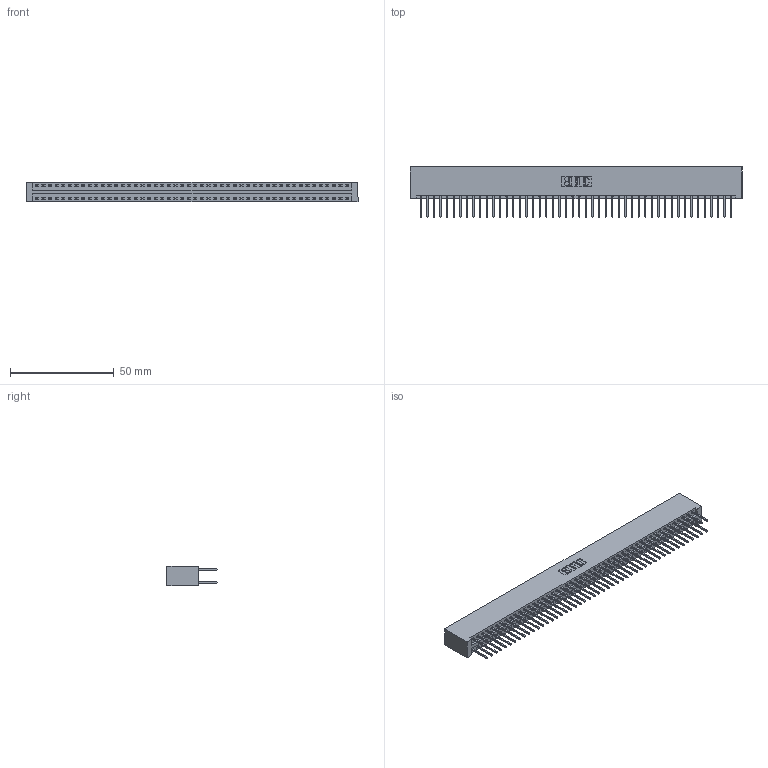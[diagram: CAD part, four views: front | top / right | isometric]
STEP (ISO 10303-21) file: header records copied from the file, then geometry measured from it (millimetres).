
FILE_DESCRIPTION (( 'STEP AP203' ), '1' );
FILE_NAME ('346-096-526-201.STEP', '2022-05-26T16:11:06', ( '' ), ( '' ), 'SwSTEP 2.0', 'SolidWorks 2020', '' );
FILE_SCHEMA (( 'CONFIG_CONTROL_DESIGN' ));
Length unit declared in the file: inch
Products named in the file (3): 346 Part_No Mounting Lugs; 346-096-526-201; 345-292-001_345-293-126
Assembly tree (97 placements, depth 2):
  346-096-526-201
    346 Part_No Mounting Lugs
    345-292-001_345-293-126  x96
Bounding box: 159.64 x 24.13 x 9.4 mm (x, y, z)
Volume: 16344.1 mm3; surface area: 23428.2 mm2
Topology: 97 solids, 97 shells, 5106 faces, 15185 edges, 9994 vertices
Faces by surface type: plane 3432, cylinder 1674
Entity records: 30259 total; most frequent: CARTESIAN_POINT 4976, ORIENTED_EDGE 4910, DIRECTION 4431, EDGE_CURVE 2455, LINE 2139, VECTOR 2139, VERTEX_POINT 1634, AXIS2_PLACEMENT_3D 1146
